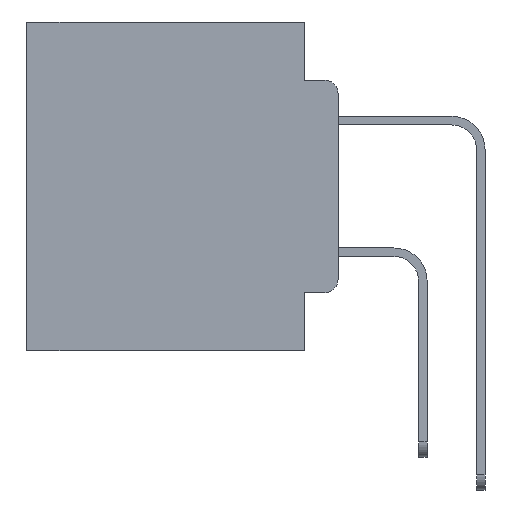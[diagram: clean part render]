
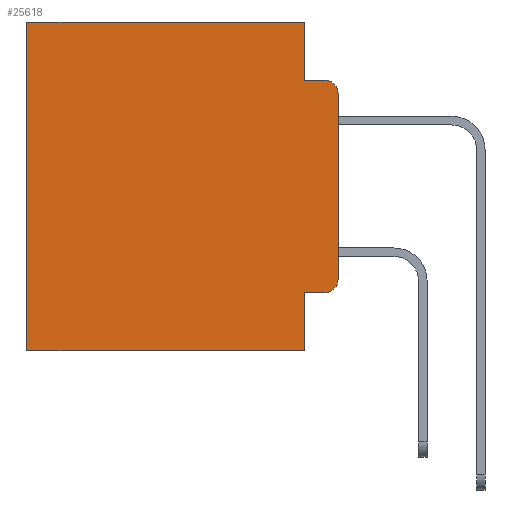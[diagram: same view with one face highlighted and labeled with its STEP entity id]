
A CAD part, left-side view. The second image highlights one B-rep face of the part: STEP entity #25618.
In plain terms, the highlighted planar face has unit normal (-1, 0, 0).
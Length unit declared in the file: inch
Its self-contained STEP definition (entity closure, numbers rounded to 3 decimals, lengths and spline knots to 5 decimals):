
#47 = CARTESIAN_POINT ( 'NONE',  ( 0.298, 0., 0. ) ) ;
#192 = CIRCLE ( 'NONE', #22390, 0.02 ) ;
#966 = AXIS2_PLACEMENT_3D ( 'NONE', #22509, #24867, #10681 ) ;
#1205 = CARTESIAN_POINT ( 'NONE',  ( 0.298, 0.02, -0.1085 ) ) ;
#1246 = LINE ( 'NONE', #17541, #13102 ) ;
#1686 = CIRCLE ( 'NONE', #10562, 0.02 ) ;
#1925 = ORIENTED_EDGE ( 'NONE', *, *, #17957, .F. ) ;
#2279 = CARTESIAN_POINT ( 'NONE',  ( 0.298, 0.051, -0.4115 ) ) ;
#2425 = DIRECTION ( 'NONE',  ( 0., 1., 0. ) ) ;
#2663 = CARTESIAN_POINT ( 'NONE',  ( 0.298, 0.473, 0. ) ) ;
#3429 = ORIENTED_EDGE ( 'NONE', *, *, #10038, .F. ) ;
#3431 = CARTESIAN_POINT ( 'NONE',  ( 0.298, 0.02, -0.0885 ) ) ;
#3449 = CARTESIAN_POINT ( 'NONE',  ( 0.298, 0.051, -0.4115 ) ) ;
#3607 = DIRECTION ( 'NONE',  ( 0., 0., -1. ) ) ;
#3754 = EDGE_CURVE ( 'NONE', #21835, #18578, #27721, .T. ) ;
#3782 = CARTESIAN_POINT ( 'NONE',  ( 0.298, 0.051, 0. ) ) ;
#3852 = VERTEX_POINT ( 'NONE', #3431 ) ;
#3929 = LINE ( 'NONE', #20828, #28236 ) ;
#4297 = DIRECTION ( 'NONE',  ( 0., -1., 0. ) ) ;
#4654 = CARTESIAN_POINT ( 'NONE',  ( 0.298, 0.473, -0.5 ) ) ;
#4762 = VERTEX_POINT ( 'NONE', #4654 ) ;
#5579 = VERTEX_POINT ( 'NONE', #10127 ) ;
#5620 = DIRECTION ( 'NONE',  ( 0., 0., -1. ) ) ;
#6406 = ORIENTED_EDGE ( 'NONE', *, *, #28039, .T. ) ;
#7988 = VERTEX_POINT ( 'NONE', #10547 ) ;
#8233 = CARTESIAN_POINT ( 'NONE',  ( 0.298, 0., -0.5 ) ) ;
#8594 = ORIENTED_EDGE ( 'NONE', *, *, #20211, .F. ) ;
#8915 = EDGE_LOOP ( 'NONE', ( #1925, #20821, #3429, #9682, #10428, #6406, #12699, #8594, #10062, #16437 ) ) ;
#9097 = CARTESIAN_POINT ( 'NONE',  ( 0.298, 0.051, -0.0885 ) ) ;
#9682 = ORIENTED_EDGE ( 'NONE', *, *, #3754, .F. ) ;
#10038 = EDGE_CURVE ( 'NONE', #18578, #3852, #3929, .T. ) ;
#10062 = ORIENTED_EDGE ( 'NONE', *, *, #18647, .T. ) ;
#10127 = CARTESIAN_POINT ( 'NONE',  ( 0.298, 0.02, -0.4115 ) ) ;
#10428 = ORIENTED_EDGE ( 'NONE', *, *, #25339, .T. ) ;
#10547 = CARTESIAN_POINT ( 'NONE',  ( 0.298, 0., -0.3915 ) ) ;
#10562 = AXIS2_PLACEMENT_3D ( 'NONE', #1205, #17829, #3607 ) ;
#10681 = DIRECTION ( 'NONE',  ( 0., 0., -1. ) ) ;
#12699 = ORIENTED_EDGE ( 'NONE', *, *, #26866, .F. ) ;
#13067 = CARTESIAN_POINT ( 'NONE',  ( 0.298, 0.02, -0.3915 ) ) ;
#13102 = VECTOR ( 'NONE', #19872, 39.37008 ) ;
#13597 = VERTEX_POINT ( 'NONE', #21550 ) ;
#13849 = EDGE_CURVE ( 'NONE', #5579, #7988, #192, .T. ) ;
#14012 = LINE ( 'NONE', #47, #19557 ) ;
#15356 = LINE ( 'NONE', #3782, #27853 ) ;
#15460 = DIRECTION ( 'NONE',  ( 0., 0., -1. ) ) ;
#15990 = CARTESIAN_POINT ( 'NONE',  ( 0.298, 0.051, 0. ) ) ;
#16437 = ORIENTED_EDGE ( 'NONE', *, *, #13849, .T. ) ;
#16516 = DIRECTION ( 'NONE',  ( 0., -1., 0. ) ) ;
#16556 = LINE ( 'NONE', #8233, #28246 ) ;
#16607 = VECTOR ( 'NONE', #16516, 39.37008 ) ;
#16611 = DIRECTION ( 'NONE',  ( 0., 0., -1. ) ) ;
#17541 = CARTESIAN_POINT ( 'NONE',  ( 0.298, 0.473, 0. ) ) ;
#17829 = DIRECTION ( 'NONE',  ( -1., 0., 0. ) ) ;
#17957 = EDGE_CURVE ( 'NONE', #13597, #7988, #25142, .T. ) ;
#18578 = VERTEX_POINT ( 'NONE', #9097 ) ;
#18647 = EDGE_CURVE ( 'NONE', #30111, #5579, #22851, .T. ) ;
#19557 = VECTOR ( 'NONE', #2425, 39.37008 ) ;
#19603 = EDGE_CURVE ( 'NONE', #13597, #3852, #1686, .T. ) ;
#19786 = CARTESIAN_POINT ( 'NONE',  ( 0.298, 0.051, 0. ) ) ;
#19872 = DIRECTION ( 'NONE',  ( 0., 0., -1. ) ) ;
#20136 = PLANE ( 'NONE',  #966 ) ;
#20211 = EDGE_CURVE ( 'NONE', #30111, #22491, #15356, .T. ) ;
#20335 = DIRECTION ( 'NONE',  ( 0., 0., -1. ) ) ;
#20821 = ORIENTED_EDGE ( 'NONE', *, *, #19603, .T. ) ;
#20828 = CARTESIAN_POINT ( 'NONE',  ( 0.298, 0.051, -0.0885 ) ) ;
#21550 = CARTESIAN_POINT ( 'NONE',  ( 0.298, 0., -0.1085 ) ) ;
#21835 = VERTEX_POINT ( 'NONE', #15990 ) ;
#22390 = AXIS2_PLACEMENT_3D ( 'NONE', #13067, #29456, #15460 ) ;
#22491 = VERTEX_POINT ( 'NONE', #27851 ) ;
#22509 = CARTESIAN_POINT ( 'NONE',  ( 0.298, 0., 0. ) ) ;
#22851 = LINE ( 'NONE', #2279, #16607 ) ;
#22983 = VECTOR ( 'NONE', #5620, 39.37008 ) ;
#23672 = VECTOR ( 'NONE', #16611, 39.37008 ) ;
#24773 = VERTEX_POINT ( 'NONE', #2663 ) ;
#24798 = DIRECTION ( 'NONE',  ( 0., 1., 0. ) ) ;
#24867 = DIRECTION ( 'NONE',  ( 1., 0., 0. ) ) ;
#25142 = LINE ( 'NONE', #28252, #23672 ) ;
#25339 = EDGE_CURVE ( 'NONE', #21835, #24773, #14012, .T. ) ;
#25439 = FACE_OUTER_BOUND ( 'NONE', #8915, .T. ) ;
#25618 = ADVANCED_FACE ( 'NONE', ( #25439 ), #20136, .F. ) ;
#26866 = EDGE_CURVE ( 'NONE', #22491, #4762, #16556, .T. ) ;
#27721 = LINE ( 'NONE', #19786, #22983 ) ;
#27851 = CARTESIAN_POINT ( 'NONE',  ( 0.298, 0.051, -0.5 ) ) ;
#27853 = VECTOR ( 'NONE', #20335, 39.37008 ) ;
#28039 = EDGE_CURVE ( 'NONE', #24773, #4762, #1246, .T. ) ;
#28236 = VECTOR ( 'NONE', #4297, 39.37008 ) ;
#28246 = VECTOR ( 'NONE', #24798, 39.37008 ) ;
#28252 = CARTESIAN_POINT ( 'NONE',  ( 0.298, 0., 0. ) ) ;
#29456 = DIRECTION ( 'NONE',  ( -1., 0., 0. ) ) ;
#30111 = VERTEX_POINT ( 'NONE', #3449 ) ;
